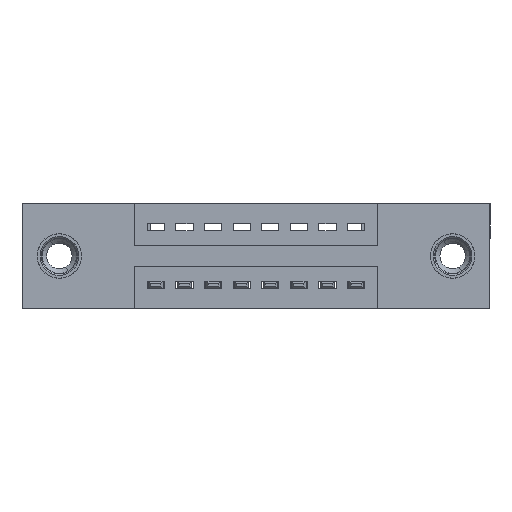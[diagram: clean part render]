
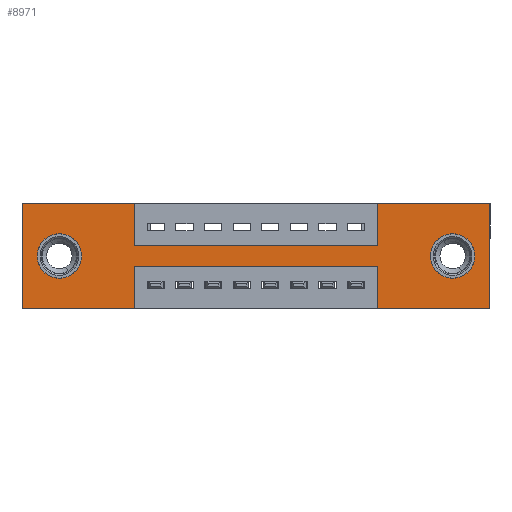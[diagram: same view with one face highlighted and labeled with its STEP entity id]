
A CAD part, front view. The second image highlights one B-rep face of the part: STEP entity #8971.
In plain terms, the highlighted planar face has unit normal (0, -1, 0).
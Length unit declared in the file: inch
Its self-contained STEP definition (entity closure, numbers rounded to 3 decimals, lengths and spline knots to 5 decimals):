
#22 = PLANE ( 'NONE',  #6134 ) ;
#44 = ORIENTED_EDGE ( 'NONE', *, *, #5802, .F. ) ;
#218 = VECTOR ( 'NONE', #2635, 39.37008 ) ;
#311 = FACE_BOUND ( 'NONE', #9736, .T. ) ;
#367 = VECTOR ( 'NONE', #1623, 39.37008 ) ;
#442 = CARTESIAN_POINT ( 'NONE',  ( 1.2425, 0., -0.15 ) ) ;
#502 = VERTEX_POINT ( 'NONE', #4977 ) ;
#543 = CARTESIAN_POINT ( 'NONE',  ( 1.635, 0., 0. ) ) ;
#555 = VECTOR ( 'NONE', #4786, 39.37008 ) ;
#594 = VECTOR ( 'NONE', #5929, 39.37008 ) ;
#639 = EDGE_CURVE ( 'NONE', #10405, #5808, #8707, .T. ) ;
#872 = VECTOR ( 'NONE', #1635, 39.37008 ) ;
#1106 = DIRECTION ( 'NONE',  ( -1., 0., 0. ) ) ;
#1314 = VERTEX_POINT ( 'NONE', #6928 ) ;
#1495 = DIRECTION ( 'NONE',  ( 0., 0., -1. ) ) ;
#1623 = DIRECTION ( 'NONE',  ( 1., 0., 0. ) ) ;
#1635 = DIRECTION ( 'NONE',  ( 0., 0., 1. ) ) ;
#1833 = DIRECTION ( 'NONE',  ( 0., 0., -1. ) ) ;
#1869 = LINE ( 'NONE', #10377, #6144 ) ;
#1886 = CARTESIAN_POINT ( 'NONE',  ( 0.3925, 0., -0.37 ) ) ;
#2008 = DIRECTION ( 'NONE',  ( 0., 0., 1. ) ) ;
#2053 = DIRECTION ( 'NONE',  ( 0., 1., 0. ) ) ;
#2149 = VECTOR ( 'NONE', #4315, 39.37008 ) ;
#2288 = AXIS2_PLACEMENT_3D ( 'NONE', #3957, #2053, #2008 ) ;
#2404 = CIRCLE ( 'NONE', #11679, 0.078 ) ;
#2475 = ORIENTED_EDGE ( 'NONE', *, *, #5002, .T. ) ;
#2482 = ORIENTED_EDGE ( 'NONE', *, *, #5654, .F. ) ;
#2618 = EDGE_CURVE ( 'NONE', #4189, #7519, #8513, .T. ) ;
#2633 = ORIENTED_EDGE ( 'NONE', *, *, #7976, .F. ) ;
#2635 = DIRECTION ( 'NONE',  ( 1., 0., 0. ) ) ;
#2707 = CARTESIAN_POINT ( 'NONE',  ( 1.505, 0., -0.107 ) ) ;
#2720 = VERTEX_POINT ( 'NONE', #442 ) ;
#2809 = ORIENTED_EDGE ( 'NONE', *, *, #2618, .F. ) ;
#2901 = DIRECTION ( 'NONE',  ( 0., -1., 0. ) ) ;
#3012 = CARTESIAN_POINT ( 'NONE',  ( 0., 0., 0. ) ) ;
#3056 = CARTESIAN_POINT ( 'NONE',  ( 1.505, 0., -0.263 ) ) ;
#3094 = ORIENTED_EDGE ( 'NONE', *, *, #3765, .F. ) ;
#3191 = ORIENTED_EDGE ( 'NONE', *, *, #3562, .F. ) ;
#3211 = VERTEX_POINT ( 'NONE', #9013 ) ;
#3372 = CARTESIAN_POINT ( 'NONE',  ( 0., 0., -0.37 ) ) ;
#3468 = LINE ( 'NONE', #5710, #872 ) ;
#3536 = EDGE_CURVE ( 'NONE', #3211, #1314, #6658, .T. ) ;
#3562 = EDGE_CURVE ( 'NONE', #5790, #9026, #3468, .T. ) ;
#3761 = AXIS2_PLACEMENT_3D ( 'NONE', #10505, #12381, #1833 ) ;
#3765 = EDGE_CURVE ( 'NONE', #10878, #6457, #5267, .T. ) ;
#3833 = FACE_BOUND ( 'NONE', #7450, .T. ) ;
#3859 = CARTESIAN_POINT ( 'NONE',  ( 0., 0., -0.37 ) ) ;
#3879 = LINE ( 'NONE', #9411, #218 ) ;
#3930 = ORIENTED_EDGE ( 'NONE', *, *, #6781, .F. ) ;
#3957 = CARTESIAN_POINT ( 'NONE',  ( 0.13, 0., -0.185 ) ) ;
#4189 = VERTEX_POINT ( 'NONE', #6511 ) ;
#4315 = DIRECTION ( 'NONE',  ( 0., 0., 1. ) ) ;
#4339 = DIRECTION ( 'NONE',  ( -1., 0., 0. ) ) ;
#4657 = EDGE_CURVE ( 'NONE', #5808, #2720, #3879, .T. ) ;
#4786 = DIRECTION ( 'NONE',  ( 0., 0., -1. ) ) ;
#4792 = EDGE_CURVE ( 'NONE', #9026, #10878, #1869, .T. ) ;
#4836 = LINE ( 'NONE', #3372, #6039 ) ;
#4977 = CARTESIAN_POINT ( 'NONE',  ( 1.635, 0., -0.37 ) ) ;
#5002 = EDGE_CURVE ( 'NONE', #7647, #5716, #9512, .T. ) ;
#5106 = CARTESIAN_POINT ( 'NONE',  ( 1.2425, 0., -0.22 ) ) ;
#5252 = LINE ( 'NONE', #6444, #9379 ) ;
#5267 = LINE ( 'NONE', #11660, #555 ) ;
#5285 = DIRECTION ( 'NONE',  ( 0., 1., 0. ) ) ;
#5585 = ORIENTED_EDGE ( 'NONE', *, *, #8348, .T. ) ;
#5628 = CARTESIAN_POINT ( 'NONE',  ( 0.3925, 0., -0.15 ) ) ;
#5654 = EDGE_CURVE ( 'NONE', #502, #5790, #7349, .T. ) ;
#5678 = DIRECTION ( 'NONE',  ( 0., 0., 1. ) ) ;
#5710 = CARTESIAN_POINT ( 'NONE',  ( 1.2425, 0., -0.37 ) ) ;
#5716 = VERTEX_POINT ( 'NONE', #3056 ) ;
#5790 = VERTEX_POINT ( 'NONE', #8537 ) ;
#5802 = EDGE_CURVE ( 'NONE', #7100, #10405, #7521, .T. ) ;
#5808 = VERTEX_POINT ( 'NONE', #5628 ) ;
#5929 = DIRECTION ( 'NONE',  ( 1., 0., 0. ) ) ;
#6039 = VECTOR ( 'NONE', #9070, 39.37008 ) ;
#6094 = ORIENTED_EDGE ( 'NONE', *, *, #639, .F. ) ;
#6126 = CARTESIAN_POINT ( 'NONE',  ( 1.2425, 0., 0. ) ) ;
#6134 = AXIS2_PLACEMENT_3D ( 'NONE', #3859, #2901, #10732 ) ;
#6144 = VECTOR ( 'NONE', #4339, 39.37008 ) ;
#6444 = CARTESIAN_POINT ( 'NONE',  ( 0., 0., 0. ) ) ;
#6454 = EDGE_CURVE ( 'NONE', #11980, #7100, #5252, .T. ) ;
#6457 = VERTEX_POINT ( 'NONE', #1886 ) ;
#6511 = CARTESIAN_POINT ( 'NONE',  ( 1.2425, 0., 0. ) ) ;
#6592 = CARTESIAN_POINT ( 'NONE',  ( 0.3925, 0., 0. ) ) ;
#6608 = ORIENTED_EDGE ( 'NONE', *, *, #6454, .F. ) ;
#6658 = CIRCLE ( 'NONE', #9921, 0.078 ) ;
#6781 = EDGE_CURVE ( 'NONE', #7519, #502, #9964, .T. ) ;
#6923 = CARTESIAN_POINT ( 'NONE',  ( 0., 0., -0.37 ) ) ;
#6928 = CARTESIAN_POINT ( 'NONE',  ( 0.13, 0., -0.107 ) ) ;
#7100 = VERTEX_POINT ( 'NONE', #10446 ) ;
#7282 = ORIENTED_EDGE ( 'NONE', *, *, #11250, .F. ) ;
#7349 = LINE ( 'NONE', #6923, #9945 ) ;
#7390 = DIRECTION ( 'NONE',  ( 0., 0., -1. ) ) ;
#7424 = CARTESIAN_POINT ( 'NONE',  ( 1.635, 0., 0. ) ) ;
#7450 = EDGE_LOOP ( 'NONE', ( #5585, #8525 ) ) ;
#7477 = ORIENTED_EDGE ( 'NONE', *, *, #4657, .F. ) ;
#7519 = VERTEX_POINT ( 'NONE', #543 ) ;
#7521 = LINE ( 'NONE', #12249, #367 ) ;
#7647 = VERTEX_POINT ( 'NONE', #2707 ) ;
#7976 = EDGE_CURVE ( 'NONE', #2720, #4189, #9323, .T. ) ;
#8202 = DIRECTION ( 'NONE',  ( 0., 0., -1. ) ) ;
#8209 = CARTESIAN_POINT ( 'NONE',  ( 0., 0., -0.37 ) ) ;
#8348 = EDGE_CURVE ( 'NONE', #1314, #3211, #9003, .T. ) ;
#8478 = CARTESIAN_POINT ( 'NONE',  ( 0.3925, 0., -0.22 ) ) ;
#8503 = DIRECTION ( 'NONE',  ( 0., 0., 1. ) ) ;
#8513 = LINE ( 'NONE', #3012, #594 ) ;
#8525 = ORIENTED_EDGE ( 'NONE', *, *, #3536, .T. ) ;
#8537 = CARTESIAN_POINT ( 'NONE',  ( 1.2425, 0., -0.37 ) ) ;
#8707 = LINE ( 'NONE', #6592, #10383 ) ;
#8903 = VECTOR ( 'NONE', #1495, 39.37008 ) ;
#8971 = ADVANCED_FACE ( 'NONE', ( #311, #3833, #9299 ), #22, .T. ) ;
#9003 = CIRCLE ( 'NONE', #2288, 0.078 ) ;
#9013 = CARTESIAN_POINT ( 'NONE',  ( 0.13, 0., -0.263 ) ) ;
#9026 = VERTEX_POINT ( 'NONE', #5106 ) ;
#9070 = DIRECTION ( 'NONE',  ( -1., 0., 0. ) ) ;
#9162 = CARTESIAN_POINT ( 'NONE',  ( 1.505, 0., -0.185 ) ) ;
#9299 = FACE_OUTER_BOUND ( 'NONE', #10814, .T. ) ;
#9323 = LINE ( 'NONE', #6126, #2149 ) ;
#9379 = VECTOR ( 'NONE', #5678, 39.37008 ) ;
#9397 = ORIENTED_EDGE ( 'NONE', *, *, #10629, .T. ) ;
#9411 = CARTESIAN_POINT ( 'NONE',  ( 0.3925, 0., -0.15 ) ) ;
#9512 = CIRCLE ( 'NONE', #3761, 0.078 ) ;
#9736 = EDGE_LOOP ( 'NONE', ( #2475, #9397 ) ) ;
#9921 = AXIS2_PLACEMENT_3D ( 'NONE', #10501, #12465, #8503 ) ;
#9945 = VECTOR ( 'NONE', #1106, 39.37008 ) ;
#9964 = LINE ( 'NONE', #7424, #8903 ) ;
#10216 = ORIENTED_EDGE ( 'NONE', *, *, #4792, .F. ) ;
#10377 = CARTESIAN_POINT ( 'NONE',  ( 0.3925, 0., -0.22 ) ) ;
#10383 = VECTOR ( 'NONE', #7390, 39.37008 ) ;
#10405 = VERTEX_POINT ( 'NONE', #12082 ) ;
#10446 = CARTESIAN_POINT ( 'NONE',  ( 0., 0., 0. ) ) ;
#10501 = CARTESIAN_POINT ( 'NONE',  ( 0.13, 0., -0.185 ) ) ;
#10505 = CARTESIAN_POINT ( 'NONE',  ( 1.505, 0., -0.185 ) ) ;
#10629 = EDGE_CURVE ( 'NONE', #5716, #7647, #2404, .T. ) ;
#10732 = DIRECTION ( 'NONE',  ( 0., 0., -1. ) ) ;
#10814 = EDGE_LOOP ( 'NONE', ( #3094, #10216, #3191, #2482, #3930, #2809, #2633, #7477, #6094, #44, #6608, #7282 ) ) ;
#10878 = VERTEX_POINT ( 'NONE', #8478 ) ;
#11250 = EDGE_CURVE ( 'NONE', #6457, #11980, #4836, .T. ) ;
#11660 = CARTESIAN_POINT ( 'NONE',  ( 0.3925, 0., -0.37 ) ) ;
#11679 = AXIS2_PLACEMENT_3D ( 'NONE', #9162, #5285, #8202 ) ;
#11980 = VERTEX_POINT ( 'NONE', #8209 ) ;
#12082 = CARTESIAN_POINT ( 'NONE',  ( 0.3925, 0., 0. ) ) ;
#12249 = CARTESIAN_POINT ( 'NONE',  ( 0., 0., 0. ) ) ;
#12381 = DIRECTION ( 'NONE',  ( 0., 1., 0. ) ) ;
#12465 = DIRECTION ( 'NONE',  ( 0., 1., 0. ) ) ;
